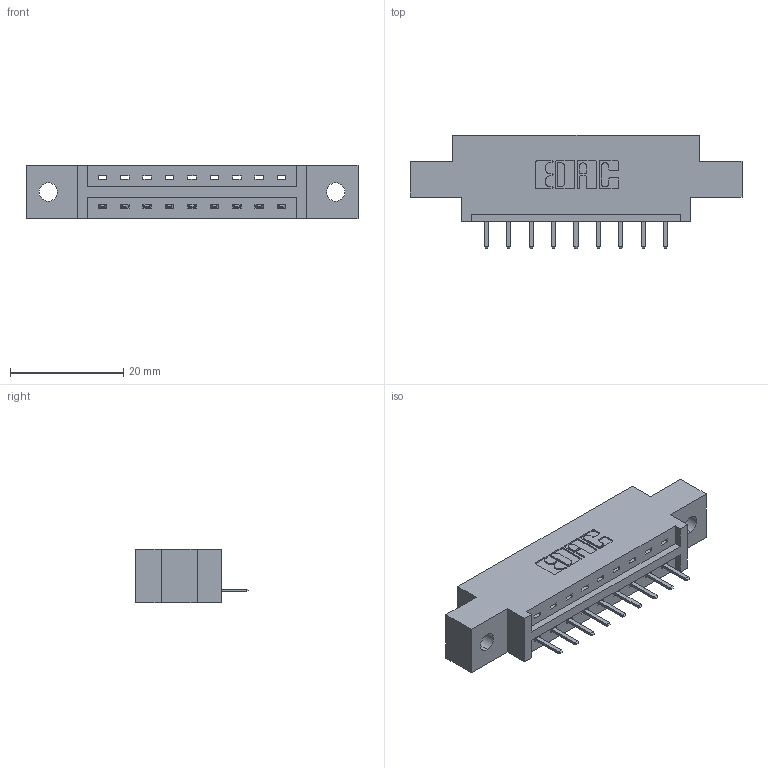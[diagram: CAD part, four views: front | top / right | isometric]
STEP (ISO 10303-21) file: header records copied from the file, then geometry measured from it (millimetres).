
FILE_DESCRIPTION (( 'STEP AP203' ), '1' );
FILE_NAME ('337-009-520-602.STEP', '2019-09-27T19:44:29', ( '' ), ( '' ), 'SwSTEP 2.0', 'SolidWorks 2016', '' );
FILE_SCHEMA (( 'CONFIG_CONTROL_DESIGN' ));
Length unit declared in the file: inch
Products named in the file (3): 337-009-520-602; 345-292-001_345-293-120; 337 Part_0.170 Offset - 0.128 Dia
Assembly tree (10 placements, depth 2):
  337-009-520-602
    337 Part_0.170 Offset - 0.128 Dia
    345-292-001_345-293-120  x9
Bounding box: 58.67 x 20.02 x 9.4 mm (x, y, z)
Volume: 5505.1 mm3; surface area: 5239 mm2
Topology: 10 solids, 10 shells, 712 faces, 2087 edges, 1366 vertices
Faces by surface type: plane 506, cylinder 206
Entity records: 11207 total; most frequent: CARTESIAN_POINT 1969, ORIENTED_EDGE 1902, DIRECTION 1713, EDGE_CURVE 951, VECTOR 819, LINE 819, VERTEX_POINT 630, AXIS2_PLACEMENT_3D 447
